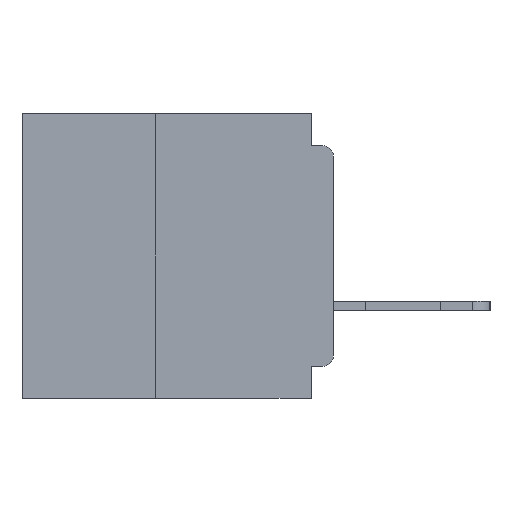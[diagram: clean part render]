
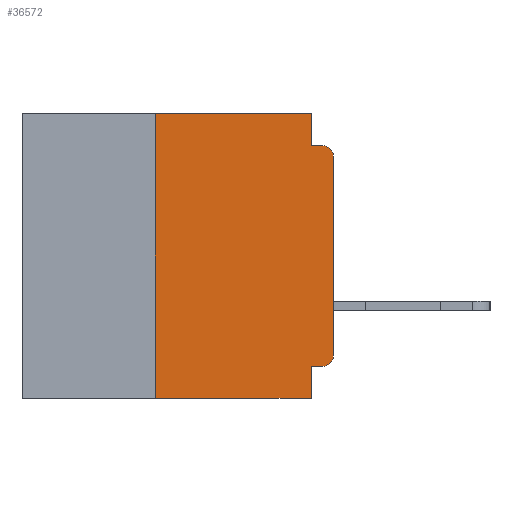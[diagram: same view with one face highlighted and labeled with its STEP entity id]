
A CAD part, left-side view. The second image highlights one B-rep face of the part: STEP entity #36572.
In plain terms, the highlighted planar face has unit normal (-1, 0, 0).
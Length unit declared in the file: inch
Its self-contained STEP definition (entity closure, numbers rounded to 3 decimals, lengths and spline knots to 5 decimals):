
#49 = DIRECTION ( 'NONE',  ( 0., 0., 1. ) ) ;
#310 = LINE ( 'NONE', #33232, #1477 ) ;
#650 = LINE ( 'NONE', #43893, #46932 ) ;
#1065 = EDGE_CURVE ( 'NONE', #24317, #5737, #44347, .T. ) ;
#1477 = VECTOR ( 'NONE', #36850, 39.37008 ) ;
#3224 = LINE ( 'NONE', #8578, #11848 ) ;
#3977 = VECTOR ( 'NONE', #34770, 39.37008 ) ;
#5737 = VERTEX_POINT ( 'NONE', #41844 ) ;
#6194 = EDGE_CURVE ( 'NONE', #5737, #14996, #6402, .T. ) ;
#6371 = VERTEX_POINT ( 'NONE', #9258 ) ;
#6402 = LINE ( 'NONE', #22939, #26002 ) ;
#7391 = EDGE_CURVE ( 'NONE', #10917, #14801, #29311, .T. ) ;
#7528 = EDGE_CURVE ( 'NONE', #13444, #12784, #33261, .T. ) ;
#7995 = CARTESIAN_POINT ( 'NONE',  ( 0., 0., -0.06 ) ) ;
#8043 = CARTESIAN_POINT ( 'NONE',  ( 0., 0.437, 0. ) ) ;
#8361 = ORIENTED_EDGE ( 'NONE', *, *, #1065, .F. ) ;
#8578 = CARTESIAN_POINT ( 'NONE',  ( 0., 0.437, 0. ) ) ;
#9046 = DIRECTION ( 'NONE',  ( -1., 0., 0. ) ) ;
#9244 = ORIENTED_EDGE ( 'NONE', *, *, #19454, .F. ) ;
#9258 = CARTESIAN_POINT ( 'NONE',  ( 0., 0.031, -0.355 ) ) ;
#10339 = ORIENTED_EDGE ( 'NONE', *, *, #43369, .F. ) ;
#10422 = VECTOR ( 'NONE', #47255, 39.37008 ) ;
#10917 = VERTEX_POINT ( 'NONE', #33132 ) ;
#11702 = DIRECTION ( 'NONE',  ( 0., 0., -1. ) ) ;
#11848 = VECTOR ( 'NONE', #23201, 39.37008 ) ;
#12334 = CARTESIAN_POINT ( 'NONE',  ( 0., 0.015, -0.34 ) ) ;
#12784 = VERTEX_POINT ( 'NONE', #19234 ) ;
#13444 = VERTEX_POINT ( 'NONE', #46618 ) ;
#14105 = AXIS2_PLACEMENT_3D ( 'NONE', #31015, #9046, #34651 ) ;
#14801 = VERTEX_POINT ( 'NONE', #18459 ) ;
#14996 = VERTEX_POINT ( 'NONE', #30436 ) ;
#16076 = DIRECTION ( 'NONE',  ( 0., 0., -1. ) ) ;
#16115 = EDGE_LOOP ( 'NONE', ( #21627, #34090, #47037, #8361, #23407, #35476, #39413, #10339, #9244, #19288 ) ) ;
#18141 = VERTEX_POINT ( 'NONE', #7995 ) ;
#18459 = CARTESIAN_POINT ( 'NONE',  ( 0., 0., -0.34 ) ) ;
#19100 = AXIS2_PLACEMENT_3D ( 'NONE', #8043, #33669, #11702 ) ;
#19234 = CARTESIAN_POINT ( 'NONE',  ( 0., 0.031, -0.4 ) ) ;
#19288 = ORIENTED_EDGE ( 'NONE', *, *, #7391, .T. ) ;
#19454 = EDGE_CURVE ( 'NONE', #10917, #6371, #29967, .T. ) ;
#19746 = EDGE_CURVE ( 'NONE', #18141, #14996, #34813, .T. ) ;
#20709 = DIRECTION ( 'NONE',  ( 0., 0., -1. ) ) ;
#21478 = CARTESIAN_POINT ( 'NONE',  ( 0., 0.031, 0. ) ) ;
#21627 = ORIENTED_EDGE ( 'NONE', *, *, #47004, .T. ) ;
#21930 = EDGE_CURVE ( 'NONE', #13444, #31556, #650, .T. ) ;
#21987 = CARTESIAN_POINT ( 'NONE',  ( 0., 0.031, 0. ) ) ;
#22624 = DIRECTION ( 'NONE',  ( 0., -1., 0. ) ) ;
#22939 = CARTESIAN_POINT ( 'NONE',  ( 0., 0., -0.045 ) ) ;
#23201 = DIRECTION ( 'NONE',  ( 0., -1., 0. ) ) ;
#23407 = ORIENTED_EDGE ( 'NONE', *, *, #47152, .F. ) ;
#24317 = VERTEX_POINT ( 'NONE', #21987 ) ;
#25107 = VECTOR ( 'NONE', #20709, 39.37008 ) ;
#26002 = VECTOR ( 'NONE', #22624, 39.37008 ) ;
#27504 = CARTESIAN_POINT ( 'NONE',  ( 0., 0.031, -0.4 ) ) ;
#29151 = CARTESIAN_POINT ( 'NONE',  ( 0., 0., -0.355 ) ) ;
#29189 = FACE_OUTER_BOUND ( 'NONE', #16115, .T. ) ;
#29311 = CIRCLE ( 'NONE', #35502, 0.015 ) ;
#29622 = VECTOR ( 'NONE', #38395, 39.37008 ) ;
#29967 = LINE ( 'NONE', #29151, #10422 ) ;
#30436 = CARTESIAN_POINT ( 'NONE',  ( 0., 0.015, -0.045 ) ) ;
#31015 = CARTESIAN_POINT ( 'NONE',  ( 0., 0.015, -0.06 ) ) ;
#31556 = VERTEX_POINT ( 'NONE', #43015 ) ;
#33132 = CARTESIAN_POINT ( 'NONE',  ( 0., 0.015, -0.355 ) ) ;
#33232 = CARTESIAN_POINT ( 'NONE',  ( 0., 0., 0. ) ) ;
#33261 = LINE ( 'NONE', #38215, #3977 ) ;
#33514 = PLANE ( 'NONE',  #19100 ) ;
#33669 = DIRECTION ( 'NONE',  ( 1., 0., 0. ) ) ;
#34090 = ORIENTED_EDGE ( 'NONE', *, *, #19746, .T. ) ;
#34651 = DIRECTION ( 'NONE',  ( 0., 0., -1. ) ) ;
#34770 = DIRECTION ( 'NONE',  ( 0., -1., 0. ) ) ;
#34813 = CIRCLE ( 'NONE', #14105, 0.015 ) ;
#35476 = ORIENTED_EDGE ( 'NONE', *, *, #21930, .F. ) ;
#35502 = AXIS2_PLACEMENT_3D ( 'NONE', #12334, #37913, #16076 ) ;
#36572 = ADVANCED_FACE ( 'NONE', ( #29189 ), #33514, .F. ) ;
#36850 = DIRECTION ( 'NONE',  ( 0., 0., 1. ) ) ;
#37913 = DIRECTION ( 'NONE',  ( -1., 0., 0. ) ) ;
#38215 = CARTESIAN_POINT ( 'NONE',  ( 0., 0.437, -0.4 ) ) ;
#38395 = DIRECTION ( 'NONE',  ( 0., 0., -1. ) ) ;
#39184 = LINE ( 'NONE', #27504, #29622 ) ;
#39413 = ORIENTED_EDGE ( 'NONE', *, *, #7528, .T. ) ;
#41844 = CARTESIAN_POINT ( 'NONE',  ( 0., 0.031, -0.045 ) ) ;
#43015 = CARTESIAN_POINT ( 'NONE',  ( 0., 0.25, 0. ) ) ;
#43369 = EDGE_CURVE ( 'NONE', #6371, #12784, #39184, .T. ) ;
#43893 = CARTESIAN_POINT ( 'NONE',  ( 0., 0.25, -0.4 ) ) ;
#44347 = LINE ( 'NONE', #21478, #25107 ) ;
#46618 = CARTESIAN_POINT ( 'NONE',  ( 0., 0.25, -0.4 ) ) ;
#46932 = VECTOR ( 'NONE', #49, 39.37008 ) ;
#47004 = EDGE_CURVE ( 'NONE', #14801, #18141, #310, .T. ) ;
#47037 = ORIENTED_EDGE ( 'NONE', *, *, #6194, .F. ) ;
#47152 = EDGE_CURVE ( 'NONE', #31556, #24317, #3224, .T. ) ;
#47255 = DIRECTION ( 'NONE',  ( 0., 1., 0. ) ) ;
